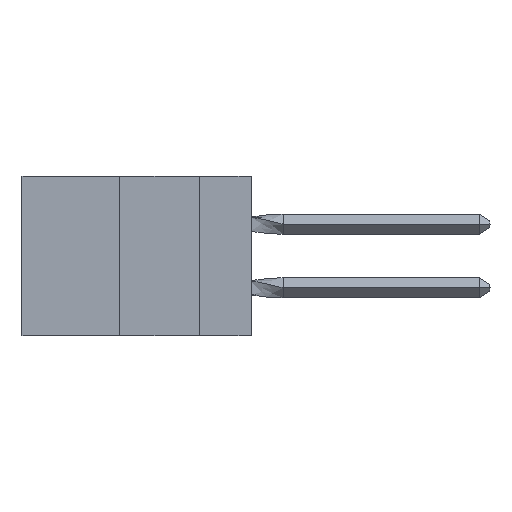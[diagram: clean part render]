
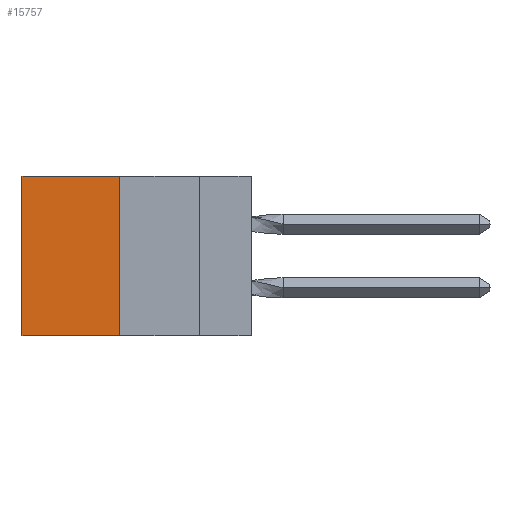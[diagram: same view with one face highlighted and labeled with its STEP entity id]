
A CAD part, left-side view. The second image highlights one B-rep face of the part: STEP entity #15757.
In plain terms, the highlighted planar face has unit normal (-1, 0, 0).
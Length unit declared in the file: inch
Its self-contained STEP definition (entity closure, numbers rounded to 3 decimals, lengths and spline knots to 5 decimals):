
#40 = VERTEX_POINT ( 'NONE', #23955 ) ;
#267 = VERTEX_POINT ( 'NONE', #12777 ) ;
#1719 = CARTESIAN_POINT ( 'NONE',  ( 0.305, 0.413, -0.5 ) ) ;
#1979 = FACE_OUTER_BOUND ( 'NONE', #18357, .T. ) ;
#3266 = VECTOR ( 'NONE', #16887, 39.37008 ) ;
#3348 = ORIENTED_EDGE ( 'NONE', *, *, #24537, .F. ) ;
#3615 = DIRECTION ( 'NONE',  ( 1., 0., 0. ) ) ;
#4660 = ORIENTED_EDGE ( 'NONE', *, *, #21783, .T. ) ;
#4905 = CARTESIAN_POINT ( 'NONE',  ( 0.305, 0.72, -0.5 ) ) ;
#6281 = AXIS2_PLACEMENT_3D ( 'NONE', #1719, #3615, #9625 ) ;
#6829 = CARTESIAN_POINT ( 'NONE',  ( 0.305, 0.413, 0. ) ) ;
#7164 = CARTESIAN_POINT ( 'NONE',  ( 0.305, 0.413, 0. ) ) ;
#8689 = LINE ( 'NONE', #16801, #20552 ) ;
#9625 = DIRECTION ( 'NONE',  ( 0., 0., -1. ) ) ;
#9782 = LINE ( 'NONE', #6829, #16588 ) ;
#11498 = PLANE ( 'NONE',  #6281 ) ;
#12777 = CARTESIAN_POINT ( 'NONE',  ( 0.305, 0.72, -0.5 ) ) ;
#14040 = EDGE_CURVE ( 'NONE', #40, #267, #22901, .T. ) ;
#15072 = ORIENTED_EDGE ( 'NONE', *, *, #17446, .F. ) ;
#15757 = ADVANCED_FACE ( 'NONE', ( #1979 ), #11498, .F. ) ;
#16244 = CARTESIAN_POINT ( 'NONE',  ( 0.305, 0.413, -0.5 ) ) ;
#16588 = VECTOR ( 'NONE', #16834, 39.37008 ) ;
#16801 = CARTESIAN_POINT ( 'NONE',  ( 0.305, 0.413, -0.5 ) ) ;
#16834 = DIRECTION ( 'NONE',  ( 0., 1., 0. ) ) ;
#16887 = DIRECTION ( 'NONE',  ( 0., 0., -1. ) ) ;
#16981 = CARTESIAN_POINT ( 'NONE',  ( 0.305, 0.413, -0.5 ) ) ;
#17446 = EDGE_CURVE ( 'NONE', #24828, #267, #8689, .T. ) ;
#17734 = VECTOR ( 'NONE', #23041, 39.37008 ) ;
#18047 = ORIENTED_EDGE ( 'NONE', *, *, #14040, .T. ) ;
#18357 = EDGE_LOOP ( 'NONE', ( #18047, #15072, #3348, #4660 ) ) ;
#18982 = LINE ( 'NONE', #16981, #17734 ) ;
#20552 = VECTOR ( 'NONE', #23301, 39.37008 ) ;
#21783 = EDGE_CURVE ( 'NONE', #24153, #40, #9782, .T. ) ;
#22901 = LINE ( 'NONE', #4905, #3266 ) ;
#23041 = DIRECTION ( 'NONE',  ( 0., 0., -1. ) ) ;
#23301 = DIRECTION ( 'NONE',  ( 0., 1., 0. ) ) ;
#23955 = CARTESIAN_POINT ( 'NONE',  ( 0.305, 0.72, 0. ) ) ;
#24153 = VERTEX_POINT ( 'NONE', #7164 ) ;
#24537 = EDGE_CURVE ( 'NONE', #24153, #24828, #18982, .T. ) ;
#24828 = VERTEX_POINT ( 'NONE', #16244 ) ;
